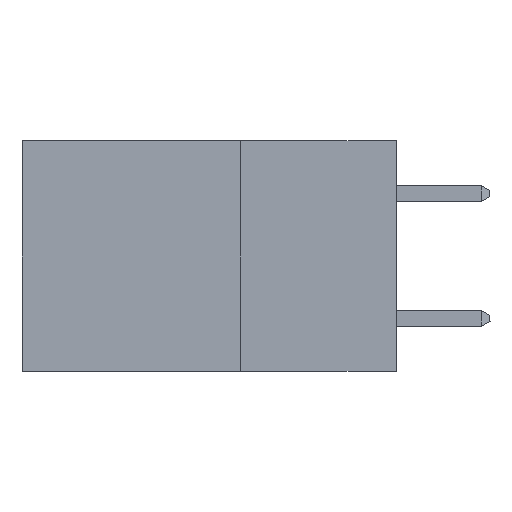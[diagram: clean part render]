
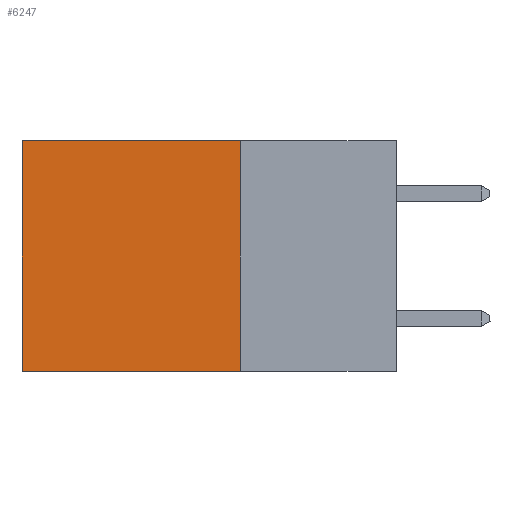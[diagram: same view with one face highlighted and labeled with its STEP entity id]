
A CAD part, left-side view. The second image highlights one B-rep face of the part: STEP entity #6247.
In plain terms, the highlighted planar face has unit normal (-1, 0, 0).
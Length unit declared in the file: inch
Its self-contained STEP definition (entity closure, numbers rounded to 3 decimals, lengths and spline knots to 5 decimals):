
#55 = CARTESIAN_POINT ( 'NONE',  ( 0.2615, 0.6, -0.37 ) ) ;
#157 = CARTESIAN_POINT ( 'NONE',  ( 0.2615, 0.25, 0. ) ) ;
#577 = ORIENTED_EDGE ( 'NONE', *, *, #20958, .F. ) ;
#936 = CARTESIAN_POINT ( 'NONE',  ( 0.2615, 0.6, -0.37 ) ) ;
#1363 = ORIENTED_EDGE ( 'NONE', *, *, #22982, .T. ) ;
#1492 = LINE ( 'NONE', #55, #12623 ) ;
#2571 = VECTOR ( 'NONE', #22045, 39.37008 ) ;
#2912 = CARTESIAN_POINT ( 'NONE',  ( 0.2615, 0.25, 0. ) ) ;
#3531 = PLANE ( 'NONE',  #8671 ) ;
#3872 = DIRECTION ( 'NONE',  ( 0., 1., 0. ) ) ;
#4952 = DIRECTION ( 'NONE',  ( 0., 1., 0. ) ) ;
#6247 = ADVANCED_FACE ( 'NONE', ( #12178 ), #3531, .F. ) ;
#6269 = LINE ( 'NONE', #2912, #16574 ) ;
#8133 = LINE ( 'NONE', #17428, #12676 ) ;
#8665 = ORIENTED_EDGE ( 'NONE', *, *, #22544, .T. ) ;
#8671 = AXIS2_PLACEMENT_3D ( 'NONE', #9521, #22919, #11454 ) ;
#9521 = CARTESIAN_POINT ( 'NONE',  ( 0.2615, 0.25, -0.37 ) ) ;
#9977 = CARTESIAN_POINT ( 'NONE',  ( 0.2615, 0.25, -0.37 ) ) ;
#11454 = DIRECTION ( 'NONE',  ( 0., 0., -1. ) ) ;
#11936 = DIRECTION ( 'NONE',  ( 0., 0., -1. ) ) ;
#12178 = FACE_OUTER_BOUND ( 'NONE', #24259, .T. ) ;
#12623 = VECTOR ( 'NONE', #11936, 39.37008 ) ;
#12676 = VECTOR ( 'NONE', #3872, 39.37008 ) ;
#13025 = LINE ( 'NONE', #20149, #2571 ) ;
#14041 = VERTEX_POINT ( 'NONE', #20592 ) ;
#14932 = VERTEX_POINT ( 'NONE', #9977 ) ;
#15680 = VERTEX_POINT ( 'NONE', #157 ) ;
#15959 = VERTEX_POINT ( 'NONE', #936 ) ;
#16313 = ORIENTED_EDGE ( 'NONE', *, *, #22055, .F. ) ;
#16574 = VECTOR ( 'NONE', #4952, 39.37008 ) ;
#17428 = CARTESIAN_POINT ( 'NONE',  ( 0.2615, 0.25, -0.37 ) ) ;
#20149 = CARTESIAN_POINT ( 'NONE',  ( 0.2615, 0.25, -0.37 ) ) ;
#20592 = CARTESIAN_POINT ( 'NONE',  ( 0.2615, 0.6, 0. ) ) ;
#20958 = EDGE_CURVE ( 'NONE', #15680, #14932, #13025, .T. ) ;
#22045 = DIRECTION ( 'NONE',  ( 0., 0., -1. ) ) ;
#22055 = EDGE_CURVE ( 'NONE', #14932, #15959, #8133, .T. ) ;
#22544 = EDGE_CURVE ( 'NONE', #15680, #14041, #6269, .T. ) ;
#22919 = DIRECTION ( 'NONE',  ( 1., 0., 0. ) ) ;
#22982 = EDGE_CURVE ( 'NONE', #14041, #15959, #1492, .T. ) ;
#24259 = EDGE_LOOP ( 'NONE', ( #1363, #16313, #577, #8665 ) ) ;
